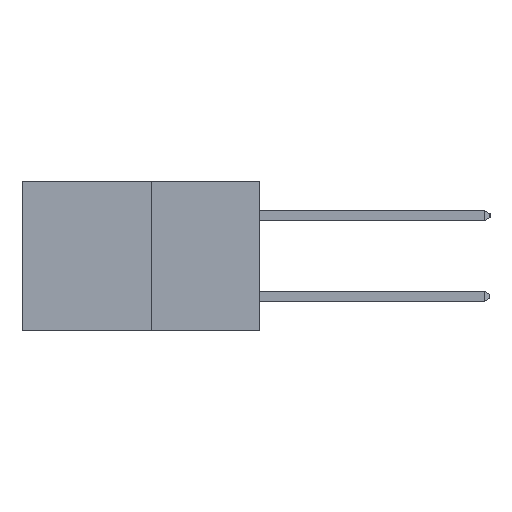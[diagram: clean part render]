
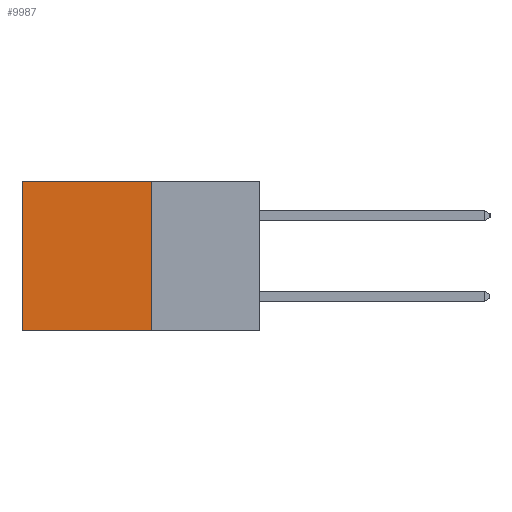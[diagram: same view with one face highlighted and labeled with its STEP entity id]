
A CAD part, left-side view. The second image highlights one B-rep face of the part: STEP entity #9987.
In plain terms, the highlighted planar face has unit normal (-1, 0, 0).
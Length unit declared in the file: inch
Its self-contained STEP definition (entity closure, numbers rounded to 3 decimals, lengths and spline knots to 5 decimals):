
#145 = DIRECTION ( 'NONE',  ( 0., 1., 0. ) ) ;
#471 = LINE ( 'NONE', #8552, #9282 ) ;
#1238 = VERTEX_POINT ( 'NONE', #1804 ) ;
#1276 = CARTESIAN_POINT ( 'NONE',  ( 0.277, 0.27, -0.37 ) ) ;
#1804 = CARTESIAN_POINT ( 'NONE',  ( 0.277, 0.27, 0. ) ) ;
#1815 = LINE ( 'NONE', #5136, #3501 ) ;
#2277 = VERTEX_POINT ( 'NONE', #1276 ) ;
#2306 = CARTESIAN_POINT ( 'NONE',  ( 0.277, 0.27, -0.37 ) ) ;
#2323 = ORIENTED_EDGE ( 'NONE', *, *, #6911, .T. ) ;
#2399 = ORIENTED_EDGE ( 'NONE', *, *, #6755, .F. ) ;
#3144 = DIRECTION ( 'NONE',  ( 1., 0., 0. ) ) ;
#3196 = DIRECTION ( 'NONE',  ( 0., 1., 0. ) ) ;
#3473 = AXIS2_PLACEMENT_3D ( 'NONE', #2306, #3144, #8591 ) ;
#3501 = VECTOR ( 'NONE', #145, 39.37008 ) ;
#3608 = EDGE_CURVE ( 'NONE', #1238, #2277, #471, .T. ) ;
#3752 = CARTESIAN_POINT ( 'NONE',  ( 0.277, 0.59, 0. ) ) ;
#4211 = VERTEX_POINT ( 'NONE', #3752 ) ;
#4412 = LINE ( 'NONE', #7984, #8498 ) ;
#5136 = CARTESIAN_POINT ( 'NONE',  ( 0.277, 0.27, 0. ) ) ;
#5415 = EDGE_LOOP ( 'NONE', ( #9285, #2399, #7834, #2323 ) ) ;
#5427 = VECTOR ( 'NONE', #8004, 39.37008 ) ;
#5735 = CARTESIAN_POINT ( 'NONE',  ( 0.277, 0.59, -0.37 ) ) ;
#6400 = CARTESIAN_POINT ( 'NONE',  ( 0.277, 0.59, -0.37 ) ) ;
#6755 = EDGE_CURVE ( 'NONE', #2277, #9858, #4412, .T. ) ;
#6911 = EDGE_CURVE ( 'NONE', #1238, #4211, #1815, .T. ) ;
#7130 = EDGE_CURVE ( 'NONE', #4211, #9858, #7779, .T. ) ;
#7277 = PLANE ( 'NONE',  #3473 ) ;
#7779 = LINE ( 'NONE', #5735, #5427 ) ;
#7834 = ORIENTED_EDGE ( 'NONE', *, *, #3608, .F. ) ;
#7984 = CARTESIAN_POINT ( 'NONE',  ( 0.277, 0.27, -0.37 ) ) ;
#8004 = DIRECTION ( 'NONE',  ( 0., 0., -1. ) ) ;
#8498 = VECTOR ( 'NONE', #3196, 39.37008 ) ;
#8538 = DIRECTION ( 'NONE',  ( 0., 0., -1. ) ) ;
#8552 = CARTESIAN_POINT ( 'NONE',  ( 0.277, 0.27, -0.37 ) ) ;
#8591 = DIRECTION ( 'NONE',  ( 0., 0., -1. ) ) ;
#9282 = VECTOR ( 'NONE', #8538, 39.37008 ) ;
#9285 = ORIENTED_EDGE ( 'NONE', *, *, #7130, .T. ) ;
#9858 = VERTEX_POINT ( 'NONE', #6400 ) ;
#9926 = FACE_OUTER_BOUND ( 'NONE', #5415, .T. ) ;
#9987 = ADVANCED_FACE ( 'NONE', ( #9926 ), #7277, .F. ) ;
